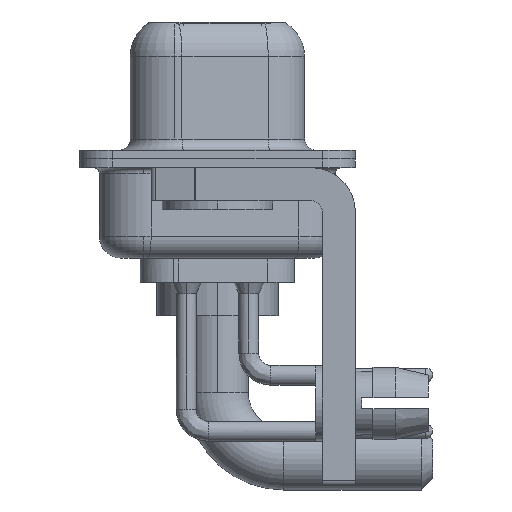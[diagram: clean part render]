
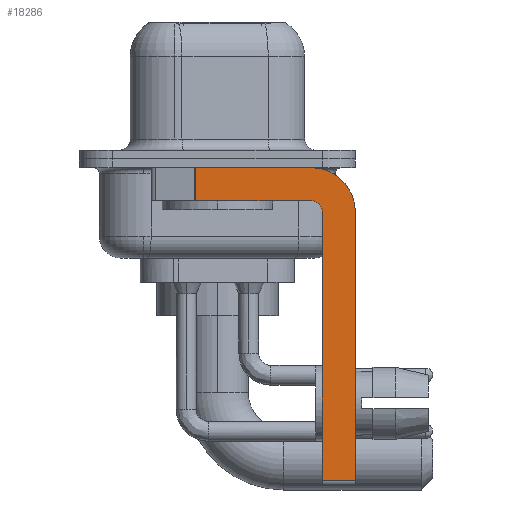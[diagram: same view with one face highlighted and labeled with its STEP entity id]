
A CAD part, left-side view. The second image highlights one B-rep face of the part: STEP entity #18286.
In plain terms, the highlighted planar face has unit normal (-1, 0, 0).
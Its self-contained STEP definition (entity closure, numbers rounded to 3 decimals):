
#355 = CARTESIAN_POINT ( 'NONE',  ( -2.9, 0.978, -1.9 ) ) ;
#431 = DIRECTION ( 'NONE',  ( 0., 1., 0. ) ) ;
#1090 = FACE_OUTER_BOUND ( 'NONE', #12022, .T. ) ;
#1673 = DIRECTION ( 'NONE',  ( 0., 0., -1. ) ) ;
#1797 = ORIENTED_EDGE ( 'NONE', *, *, #16388, .F. ) ;
#1866 = LINE ( 'NONE', #14627, #3767 ) ;
#2242 = EDGE_CURVE ( 'NONE', #13071, #15347, #1866, .T. ) ;
#2267 = DIRECTION ( 'NONE',  ( 1., 0., 0. ) ) ;
#2505 = DIRECTION ( 'NONE',  ( 1., 0., 0. ) ) ;
#2732 = CARTESIAN_POINT ( 'NONE',  ( -2.9, -4.25, -0.4 ) ) ;
#2822 = CARTESIAN_POINT ( 'NONE',  ( -2.9, 0.978, -0.4 ) ) ;
#2950 = CARTESIAN_POINT ( 'NONE',  ( -2.9, -4.75, -2.4 ) ) ;
#3103 = CARTESIAN_POINT ( 'NONE',  ( -2.9, -4.75, -14.55 ) ) ;
#3204 = DIRECTION ( 'NONE',  ( 0., 0., -1. ) ) ;
#3464 = EDGE_CURVE ( 'NONE', #5132, #17686, #12866, .T. ) ;
#3767 = VECTOR ( 'NONE', #1673, 1000. ) ;
#3892 = EDGE_CURVE ( 'NONE', #10818, #11572, #14603, .T. ) ;
#5047 = AXIS2_PLACEMENT_3D ( 'NONE', #12108, #9158, #14930 ) ;
#5119 = CARTESIAN_POINT ( 'NONE',  ( -2.9, -4.25, -1.9 ) ) ;
#5132 = VERTEX_POINT ( 'NONE', #3103 ) ;
#5328 = VERTEX_POINT ( 'NONE', #5119 ) ;
#5372 = PLANE ( 'NONE',  #7210 ) ;
#6139 = LINE ( 'NONE', #11883, #10820 ) ;
#6464 = EDGE_CURVE ( 'NONE', #10818, #18197, #10378, .T. ) ;
#6645 = DIRECTION ( 'NONE',  ( 0., 0., -1. ) ) ;
#6657 = CIRCLE ( 'NONE', #15981, 2. ) ;
#6868 = DIRECTION ( 'NONE',  ( 0., 0., -1. ) ) ;
#7210 = AXIS2_PLACEMENT_3D ( 'NONE', #9515, #2505, #6868 ) ;
#7580 = ORIENTED_EDGE ( 'NONE', *, *, #3892, .F. ) ;
#7622 = CARTESIAN_POINT ( 'NONE',  ( -2.9, -4.25, -1.9 ) ) ;
#9033 = CARTESIAN_POINT ( 'NONE',  ( -2.9, -6.25, -14.55 ) ) ;
#9158 = DIRECTION ( 'NONE',  ( -1., 0., 0. ) ) ;
#9515 = CARTESIAN_POINT ( 'NONE',  ( -2.9, -4.25, -2.4 ) ) ;
#9863 = VECTOR ( 'NONE', #3204, 1000. ) ;
#10254 = EDGE_CURVE ( 'NONE', #11572, #13071, #6657, .T. ) ;
#10378 = LINE ( 'NONE', #13611, #9863 ) ;
#10637 = LINE ( 'NONE', #7622, #13153 ) ;
#10818 = VERTEX_POINT ( 'NONE', #2822 ) ;
#10820 = VECTOR ( 'NONE', #13596, 1000. ) ;
#11381 = ORIENTED_EDGE ( 'NONE', *, *, #15387, .F. ) ;
#11572 = VERTEX_POINT ( 'NONE', #2732 ) ;
#11730 = DIRECTION ( 'NONE',  ( 0., 0., 1. ) ) ;
#11883 = CARTESIAN_POINT ( 'NONE',  ( -2.9, -4.25, -14.55 ) ) ;
#11981 = CIRCLE ( 'NONE', #5047, 0.5 ) ;
#12022 = EDGE_LOOP ( 'NONE', ( #7580, #15462, #11381, #1797, #17547, #12366, #13138, #18626 ) ) ;
#12108 = CARTESIAN_POINT ( 'NONE',  ( -2.9, -4.25, -2.4 ) ) ;
#12366 = ORIENTED_EDGE ( 'NONE', *, *, #18198, .T. ) ;
#12866 = LINE ( 'NONE', #15777, #17963 ) ;
#13071 = VERTEX_POINT ( 'NONE', #15873 ) ;
#13138 = ORIENTED_EDGE ( 'NONE', *, *, #2242, .F. ) ;
#13153 = VECTOR ( 'NONE', #431, 1000. ) ;
#13198 = DIRECTION ( 'NONE',  ( 0., -1., 0. ) ) ;
#13596 = DIRECTION ( 'NONE',  ( 0., -1., 0. ) ) ;
#13611 = CARTESIAN_POINT ( 'NONE',  ( -2.9, 0.978, -1.9 ) ) ;
#14603 = LINE ( 'NONE', #15827, #16754 ) ;
#14627 = CARTESIAN_POINT ( 'NONE',  ( -2.9, -6.25, -2.4 ) ) ;
#14930 = DIRECTION ( 'NONE',  ( 0., 0., 1. ) ) ;
#15347 = VERTEX_POINT ( 'NONE', #9033 ) ;
#15387 = EDGE_CURVE ( 'NONE', #5328, #18197, #10637, .T. ) ;
#15462 = ORIENTED_EDGE ( 'NONE', *, *, #6464, .T. ) ;
#15777 = CARTESIAN_POINT ( 'NONE',  ( -2.9, -4.75, -14.8 ) ) ;
#15827 = CARTESIAN_POINT ( 'NONE',  ( -2.9, 3., -0.4 ) ) ;
#15873 = CARTESIAN_POINT ( 'NONE',  ( -2.9, -6.25, -2.4 ) ) ;
#15981 = AXIS2_PLACEMENT_3D ( 'NONE', #16930, #2267, #6645 ) ;
#16388 = EDGE_CURVE ( 'NONE', #17686, #5328, #11981, .T. ) ;
#16754 = VECTOR ( 'NONE', #13198, 1000. ) ;
#16930 = CARTESIAN_POINT ( 'NONE',  ( -2.9, -4.25, -2.4 ) ) ;
#17547 = ORIENTED_EDGE ( 'NONE', *, *, #3464, .F. ) ;
#17686 = VERTEX_POINT ( 'NONE', #2950 ) ;
#17963 = VECTOR ( 'NONE', #11730, 1000. ) ;
#18197 = VERTEX_POINT ( 'NONE', #355 ) ;
#18198 = EDGE_CURVE ( 'NONE', #5132, #15347, #6139, .T. ) ;
#18286 = ADVANCED_FACE ( 'NONE', ( #1090 ), #5372, .F. ) ;
#18626 = ORIENTED_EDGE ( 'NONE', *, *, #10254, .F. ) ;
